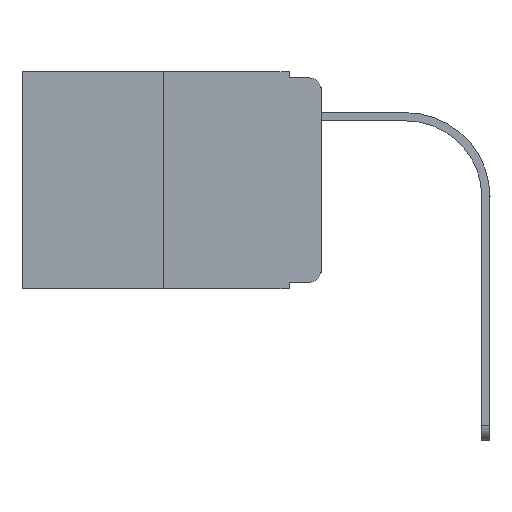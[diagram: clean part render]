
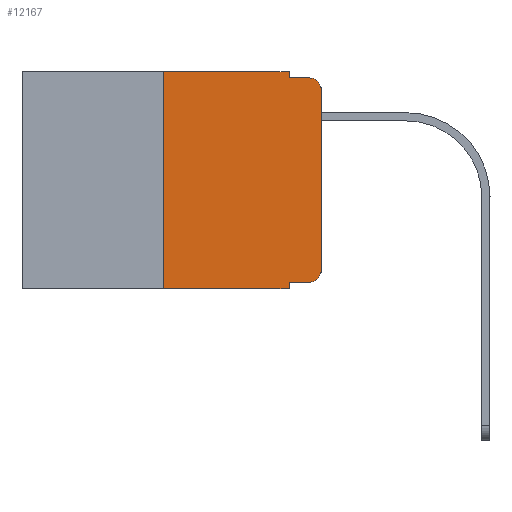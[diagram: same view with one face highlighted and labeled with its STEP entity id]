
A CAD part, left-side view. The second image highlights one B-rep face of the part: STEP entity #12167.
In plain terms, the highlighted planar face has unit normal (-1, 0, 0).
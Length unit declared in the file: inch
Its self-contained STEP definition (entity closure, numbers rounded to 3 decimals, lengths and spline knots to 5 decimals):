
#197 = CARTESIAN_POINT ( 'NONE',  ( 0., 0.02, -0.333 ) ) ;
#226 = CARTESIAN_POINT ( 'NONE',  ( 0., 0.02, -0.313 ) ) ;
#402 = AXIS2_PLACEMENT_3D ( 'NONE', #226, #10890, #21748 ) ;
#431 = ORIENTED_EDGE ( 'NONE', *, *, #17414, .T. ) ;
#481 = AXIS2_PLACEMENT_3D ( 'NONE', #23523, #14447, #8957 ) ;
#827 = VECTOR ( 'NONE', #2665, 39.37008 ) ;
#1120 = VERTEX_POINT ( 'NONE', #13983 ) ;
#1193 = EDGE_LOOP ( 'NONE', ( #431, #13964, #15309, #9534, #5156, #11060, #15200, #5616, #8199, #20868 ) ) ;
#1576 = VECTOR ( 'NONE', #6001, 39.37008 ) ;
#2216 = DIRECTION ( 'NONE',  ( 0., 0., -1. ) ) ;
#2665 = DIRECTION ( 'NONE',  ( 0., -1., 0. ) ) ;
#2699 = VERTEX_POINT ( 'NONE', #6523 ) ;
#2715 = DIRECTION ( 'NONE',  ( -1., 0., 0. ) ) ;
#3650 = DIRECTION ( 'NONE',  ( 0., 0., -1. ) ) ;
#3754 = DIRECTION ( 'NONE',  ( 0., 0., 1. ) ) ;
#3790 = CARTESIAN_POINT ( 'NONE',  ( 0., 0.051, -0.01 ) ) ;
#5156 = ORIENTED_EDGE ( 'NONE', *, *, #14904, .F. ) ;
#5312 = LINE ( 'NONE', #5668, #18391 ) ;
#5616 = ORIENTED_EDGE ( 'NONE', *, *, #6637, .F. ) ;
#5668 = CARTESIAN_POINT ( 'NONE',  ( 0., 0.051, 0. ) ) ;
#6001 = DIRECTION ( 'NONE',  ( 0., 0., -1. ) ) ;
#6175 = VECTOR ( 'NONE', #3754, 39.37008 ) ;
#6523 = CARTESIAN_POINT ( 'NONE',  ( 0., 0.25, -0.343 ) ) ;
#6533 = VECTOR ( 'NONE', #20078, 39.37008 ) ;
#6637 = EDGE_CURVE ( 'NONE', #16397, #1120, #5312, .T. ) ;
#6665 = EDGE_CURVE ( 'NONE', #2699, #7764, #11062, .T. ) ;
#6730 = LINE ( 'NONE', #12231, #13540 ) ;
#7101 = EDGE_CURVE ( 'NONE', #7746, #19611, #11749, .T. ) ;
#7417 = CARTESIAN_POINT ( 'NONE',  ( 0., 0., -0.313 ) ) ;
#7746 = VERTEX_POINT ( 'NONE', #23074 ) ;
#7764 = VERTEX_POINT ( 'NONE', #11726 ) ;
#8199 = ORIENTED_EDGE ( 'NONE', *, *, #23010, .T. ) ;
#8198 = CARTESIAN_POINT ( 'NONE',  ( 0., 0., -0.03 ) ) ;
#8733 = CARTESIAN_POINT ( 'NONE',  ( 0., 0.051, -0.01 ) ) ;
#8957 = DIRECTION ( 'NONE',  ( 0., 0., -1. ) ) ;
#9187 = PLANE ( 'NONE',  #481 ) ;
#9534 = ORIENTED_EDGE ( 'NONE', *, *, #7101, .F. ) ;
#10454 = EDGE_CURVE ( 'NONE', #10906, #10459, #13026, .T. ) ;
#10459 = VERTEX_POINT ( 'NONE', #7417 ) ;
#10890 = DIRECTION ( 'NONE',  ( -1., 0., 0. ) ) ;
#10906 = VERTEX_POINT ( 'NONE', #197 ) ;
#11060 = ORIENTED_EDGE ( 'NONE', *, *, #6665, .F. ) ;
#11062 = LINE ( 'NONE', #22165, #6175 ) ;
#11317 = CARTESIAN_POINT ( 'NONE',  ( 0., 0.051, -0.333 ) ) ;
#11516 = CARTESIAN_POINT ( 'NONE',  ( 0., 0.051, 0. ) ) ;
#11643 = EDGE_CURVE ( 'NONE', #2699, #1120, #11773, .T. ) ;
#11726 = CARTESIAN_POINT ( 'NONE',  ( 0., 0.25, 0. ) ) ;
#11749 = LINE ( 'NONE', #11516, #1576 ) ;
#11773 = LINE ( 'NONE', #19063, #827 ) ;
#12167 = ADVANCED_FACE ( 'NONE', ( #18165 ), #9187, .F. ) ;
#12231 = CARTESIAN_POINT ( 'NONE',  ( 0., 0.473, 0. ) ) ;
#12558 = EDGE_CURVE ( 'NONE', #13210, #15686, #12685, .T. ) ;
#12685 = CIRCLE ( 'NONE', #19171, 0.02 ) ;
#13026 = CIRCLE ( 'NONE', #402, 0.02 ) ;
#13210 = VERTEX_POINT ( 'NONE', #8198 ) ;
#13540 = VECTOR ( 'NONE', #19525, 39.37008 ) ;
#13964 = ORIENTED_EDGE ( 'NONE', *, *, #12558, .T. ) ;
#13983 = CARTESIAN_POINT ( 'NONE',  ( 0., 0.051, -0.343 ) ) ;
#14447 = DIRECTION ( 'NONE',  ( 1., 0., 0. ) ) ;
#14904 = EDGE_CURVE ( 'NONE', #7764, #7746, #6730, .T. ) ;
#15146 = DIRECTION ( 'NONE',  ( 0., 0., 1. ) ) ;
#15200 = ORIENTED_EDGE ( 'NONE', *, *, #11643, .T. ) ;
#15248 = LINE ( 'NONE', #11317, #19094 ) ;
#15309 = ORIENTED_EDGE ( 'NONE', *, *, #16770, .F. ) ;
#15686 = VERTEX_POINT ( 'NONE', #17102 ) ;
#16397 = VERTEX_POINT ( 'NONE', #20934 ) ;
#16633 = LINE ( 'NONE', #3790, #6533 ) ;
#16770 = EDGE_CURVE ( 'NONE', #19611, #15686, #16633, .T. ) ;
#16958 = LINE ( 'NONE', #22777, #17645 ) ;
#17102 = CARTESIAN_POINT ( 'NONE',  ( 0., 0.02, -0.01 ) ) ;
#17414 = EDGE_CURVE ( 'NONE', #10459, #13210, #16958, .T. ) ;
#17645 = VECTOR ( 'NONE', #15146, 39.37008 ) ;
#18165 = FACE_OUTER_BOUND ( 'NONE', #1193, .T. ) ;
#18391 = VECTOR ( 'NONE', #3650, 39.37008 ) ;
#19063 = CARTESIAN_POINT ( 'NONE',  ( 0., 0.473, -0.343 ) ) ;
#19094 = VECTOR ( 'NONE', #22172, 39.37008 ) ;
#19109 = CARTESIAN_POINT ( 'NONE',  ( 0., 0.02, -0.03 ) ) ;
#19171 = AXIS2_PLACEMENT_3D ( 'NONE', #19109, #2715, #2216 ) ;
#19525 = DIRECTION ( 'NONE',  ( 0., -1., 0. ) ) ;
#19611 = VERTEX_POINT ( 'NONE', #8733 ) ;
#20078 = DIRECTION ( 'NONE',  ( 0., -1., 0. ) ) ;
#20868 = ORIENTED_EDGE ( 'NONE', *, *, #10454, .T. ) ;
#20934 = CARTESIAN_POINT ( 'NONE',  ( 0., 0.051, -0.333 ) ) ;
#21748 = DIRECTION ( 'NONE',  ( 0., 0., -1. ) ) ;
#22165 = CARTESIAN_POINT ( 'NONE',  ( 0., 0.25, 0. ) ) ;
#22172 = DIRECTION ( 'NONE',  ( 0., -1., 0. ) ) ;
#22777 = CARTESIAN_POINT ( 'NONE',  ( 0., 0., 0. ) ) ;
#23010 = EDGE_CURVE ( 'NONE', #16397, #10906, #15248, .T. ) ;
#23074 = CARTESIAN_POINT ( 'NONE',  ( 0., 0.051, 0. ) ) ;
#23523 = CARTESIAN_POINT ( 'NONE',  ( 0., 0.473, 0. ) ) ;
